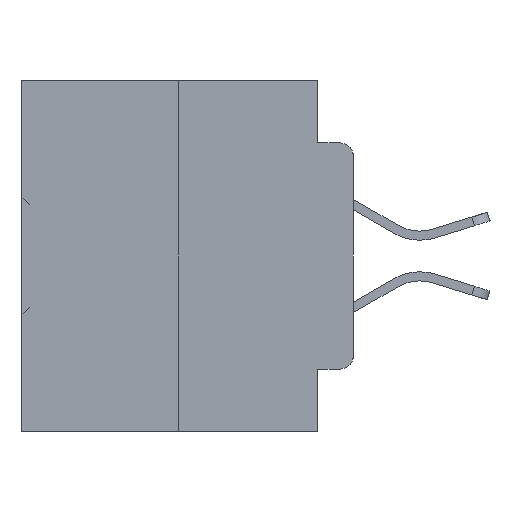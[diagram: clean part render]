
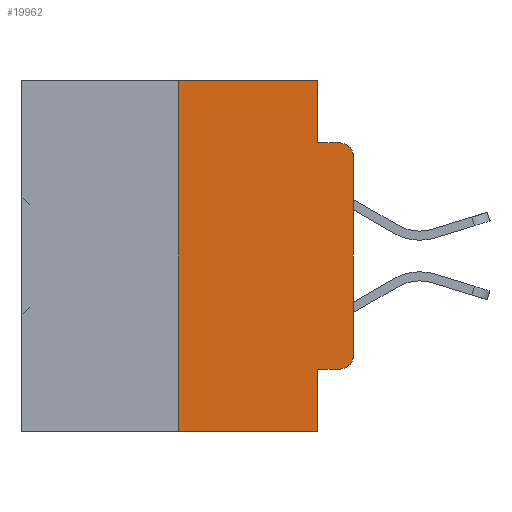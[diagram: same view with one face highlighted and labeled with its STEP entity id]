
A CAD part, left-side view. The second image highlights one B-rep face of the part: STEP entity #19962.
In plain terms, the highlighted planar face has unit normal (-1, 0, 0).
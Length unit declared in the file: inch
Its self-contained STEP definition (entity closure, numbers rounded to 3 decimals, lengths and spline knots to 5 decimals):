
#314 = VERTEX_POINT ( 'NONE', #15048 ) ;
#767 = DIRECTION ( 'NONE',  ( 0., -1., 0. ) ) ;
#1030 = EDGE_CURVE ( 'NONE', #2899, #21372, #22878, .T. ) ;
#1160 = CARTESIAN_POINT ( 'NONE',  ( 0., 0.051, 0. ) ) ;
#1383 = LINE ( 'NONE', #3928, #15063 ) ;
#1801 = CARTESIAN_POINT ( 'NONE',  ( 0., 0.25, 0. ) ) ;
#1993 = DIRECTION ( 'NONE',  ( 0., 0., 1. ) ) ;
#2522 = CARTESIAN_POINT ( 'NONE',  ( 0., 0.25, -0.5 ) ) ;
#2899 = VERTEX_POINT ( 'NONE', #27707 ) ;
#3928 = CARTESIAN_POINT ( 'NONE',  ( 0., 0.051, -0.0885 ) ) ;
#4603 = VECTOR ( 'NONE', #1993, 39.37008 ) ;
#4682 = CARTESIAN_POINT ( 'NONE',  ( 0., 0.051, 0. ) ) ;
#5417 = EDGE_CURVE ( 'NONE', #21372, #20356, #21191, .T. ) ;
#5622 = ORIENTED_EDGE ( 'NONE', *, *, #24843, .T. ) ;
#7838 = VERTEX_POINT ( 'NONE', #32107 ) ;
#8858 = CARTESIAN_POINT ( 'NONE',  ( 0., 0.02, -0.3915 ) ) ;
#8870 = VECTOR ( 'NONE', #15617, 39.37008 ) ;
#9165 = CARTESIAN_POINT ( 'NONE',  ( 0., 0.02, -0.0885 ) ) ;
#10715 = ORIENTED_EDGE ( 'NONE', *, *, #19804, .T. ) ;
#11018 = PLANE ( 'NONE',  #37458 ) ;
#11431 = EDGE_CURVE ( 'NONE', #25168, #2899, #26210, .T. ) ;
#12858 = CIRCLE ( 'NONE', #24586, 0.02 ) ;
#13165 = FACE_OUTER_BOUND ( 'NONE', #17139, .T. ) ;
#13217 = DIRECTION ( 'NONE',  ( 0., -1., 0. ) ) ;
#14166 = CARTESIAN_POINT ( 'NONE',  ( 0., 0.473, -0.5 ) ) ;
#14206 = CARTESIAN_POINT ( 'NONE',  ( 0., 0., 0. ) ) ;
#14483 = AXIS2_PLACEMENT_3D ( 'NONE', #8858, #20653, #32457 ) ;
#15048 = CARTESIAN_POINT ( 'NONE',  ( 0., 0., -0.3915 ) ) ;
#15063 = VECTOR ( 'NONE', #13217, 39.37008 ) ;
#15617 = DIRECTION ( 'NONE',  ( 0., -1., 0. ) ) ;
#15800 = VECTOR ( 'NONE', #767, 39.37008 ) ;
#17139 = EDGE_LOOP ( 'NONE', ( #5622, #28990, #17674, #36787, #29510, #22215, #10715, #29173, #17675, #25643 ) ) ;
#17674 = ORIENTED_EDGE ( 'NONE', *, *, #28827, .F. ) ;
#17675 = ORIENTED_EDGE ( 'NONE', *, *, #35674, .T. ) ;
#17982 = DIRECTION ( 'NONE',  ( 0., -1., 0. ) ) ;
#18512 = LINE ( 'NONE', #30328, #8870 ) ;
#18784 = DIRECTION ( 'NONE',  ( 0., 0., -1. ) ) ;
#19339 = DIRECTION ( 'NONE',  ( 0., 0., -1. ) ) ;
#19804 = EDGE_CURVE ( 'NONE', #25168, #29740, #29838, .T. ) ;
#19962 = ADVANCED_FACE ( 'NONE', ( #13165 ), #11018, .F. ) ;
#20356 = VERTEX_POINT ( 'NONE', #24148 ) ;
#20653 = DIRECTION ( 'NONE',  ( -1., 0., 0. ) ) ;
#20964 = VECTOR ( 'NONE', #26003, 39.37008 ) ;
#21191 = LINE ( 'NONE', #27203, #23279 ) ;
#21372 = VERTEX_POINT ( 'NONE', #4682 ) ;
#21488 = EDGE_CURVE ( 'NONE', #30667, #36691, #12858, .T. ) ;
#22067 = LINE ( 'NONE', #1160, #35206 ) ;
#22153 = CARTESIAN_POINT ( 'NONE',  ( 0., 0.051, -0.5 ) ) ;
#22215 = ORIENTED_EDGE ( 'NONE', *, *, #11431, .F. ) ;
#22878 = LINE ( 'NONE', #31985, #24934 ) ;
#23279 = VECTOR ( 'NONE', #35710, 39.37008 ) ;
#23396 = DIRECTION ( 'NONE',  ( 0., 0., -1. ) ) ;
#23585 = DIRECTION ( 'NONE',  ( -1., 0., 0. ) ) ;
#24148 = CARTESIAN_POINT ( 'NONE',  ( 0., 0.051, -0.0885 ) ) ;
#24586 = AXIS2_PLACEMENT_3D ( 'NONE', #32508, #23585, #23396 ) ;
#24843 = EDGE_CURVE ( 'NONE', #314, #30667, #31615, .T. ) ;
#24934 = VECTOR ( 'NONE', #17982, 39.37008 ) ;
#25168 = VERTEX_POINT ( 'NONE', #2522 ) ;
#25643 = ORIENTED_EDGE ( 'NONE', *, *, #29505, .T. ) ;
#26003 = DIRECTION ( 'NONE',  ( 0., 0., 1. ) ) ;
#26210 = LINE ( 'NONE', #1801, #4603 ) ;
#26218 = CIRCLE ( 'NONE', #14483, 0.02 ) ;
#27203 = CARTESIAN_POINT ( 'NONE',  ( 0., 0.051, 0. ) ) ;
#27571 = CARTESIAN_POINT ( 'NONE',  ( 0., 0.051, -0.4115 ) ) ;
#27707 = CARTESIAN_POINT ( 'NONE',  ( 0., 0.25, 0. ) ) ;
#28061 = CARTESIAN_POINT ( 'NONE',  ( 0., 0.473, 0. ) ) ;
#28827 = EDGE_CURVE ( 'NONE', #20356, #36691, #1383, .T. ) ;
#28990 = ORIENTED_EDGE ( 'NONE', *, *, #21488, .T. ) ;
#29173 = ORIENTED_EDGE ( 'NONE', *, *, #30623, .F. ) ;
#29505 = EDGE_CURVE ( 'NONE', #7838, #314, #26218, .T. ) ;
#29510 = ORIENTED_EDGE ( 'NONE', *, *, #1030, .F. ) ;
#29740 = VERTEX_POINT ( 'NONE', #22153 ) ;
#29838 = LINE ( 'NONE', #14166, #15800 ) ;
#30328 = CARTESIAN_POINT ( 'NONE',  ( 0., 0.051, -0.4115 ) ) ;
#30623 = EDGE_CURVE ( 'NONE', #36210, #29740, #22067, .T. ) ;
#30667 = VERTEX_POINT ( 'NONE', #36201 ) ;
#31615 = LINE ( 'NONE', #14206, #20964 ) ;
#31985 = CARTESIAN_POINT ( 'NONE',  ( 0., 0.473, 0. ) ) ;
#32107 = CARTESIAN_POINT ( 'NONE',  ( 0., 0.02, -0.4115 ) ) ;
#32457 = DIRECTION ( 'NONE',  ( 0., 0., -1. ) ) ;
#32508 = CARTESIAN_POINT ( 'NONE',  ( 0., 0.02, -0.1085 ) ) ;
#35206 = VECTOR ( 'NONE', #18784, 39.37008 ) ;
#35674 = EDGE_CURVE ( 'NONE', #36210, #7838, #18512, .T. ) ;
#35710 = DIRECTION ( 'NONE',  ( 0., 0., -1. ) ) ;
#36201 = CARTESIAN_POINT ( 'NONE',  ( 0., 0., -0.1085 ) ) ;
#36210 = VERTEX_POINT ( 'NONE', #27571 ) ;
#36691 = VERTEX_POINT ( 'NONE', #9165 ) ;
#36763 = DIRECTION ( 'NONE',  ( 1., 0., 0. ) ) ;
#36787 = ORIENTED_EDGE ( 'NONE', *, *, #5417, .F. ) ;
#37458 = AXIS2_PLACEMENT_3D ( 'NONE', #28061, #36763, #19339 ) ;
